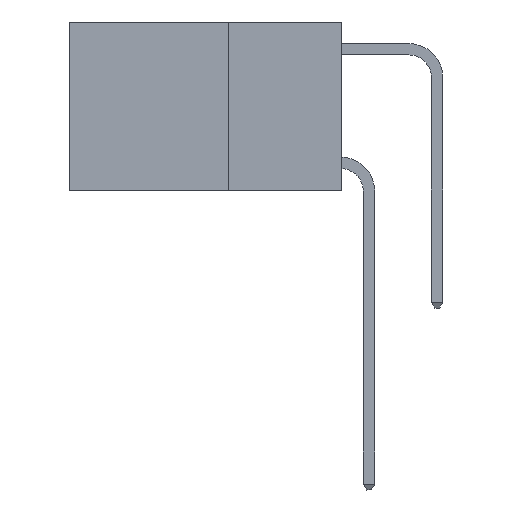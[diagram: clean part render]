
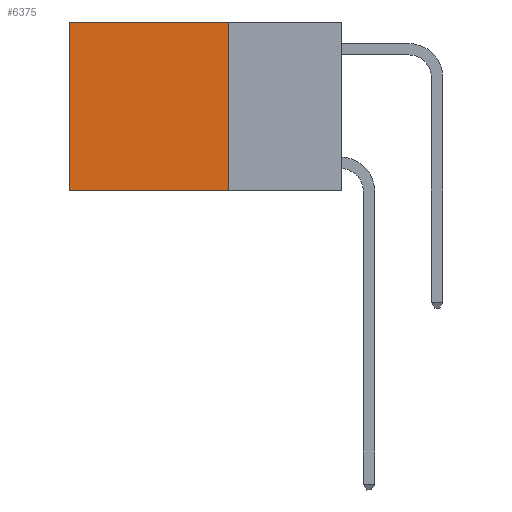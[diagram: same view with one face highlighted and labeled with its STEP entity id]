
A CAD part, left-side view. The second image highlights one B-rep face of the part: STEP entity #6375.
In plain terms, the highlighted planar face has unit normal (-1, 0, 0).
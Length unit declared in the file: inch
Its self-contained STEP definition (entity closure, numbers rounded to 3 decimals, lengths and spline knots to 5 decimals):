
#297 = CARTESIAN_POINT ( 'NONE',  ( 0.2625, 0.25, 0. ) ) ;
#798 = EDGE_CURVE ( 'NONE', #8440, #4409, #9333, .T. ) ;
#1024 = LINE ( 'NONE', #9739, #7808 ) ;
#1093 = DIRECTION ( 'NONE',  ( 0., 0., -1. ) ) ;
#1301 = DIRECTION ( 'NONE',  ( 1., 0., 0. ) ) ;
#1322 = LINE ( 'NONE', #11291, #12889 ) ;
#1547 = ORIENTED_EDGE ( 'NONE', *, *, #3289, .F. ) ;
#1710 = EDGE_LOOP ( 'NONE', ( #4981, #1547, #9969, #10829 ) ) ;
#3289 = EDGE_CURVE ( 'NONE', #4409, #6007, #1322, .T. ) ;
#3851 = DIRECTION ( 'NONE',  ( 0., 0., -1. ) ) ;
#3880 = LINE ( 'NONE', #4791, #10066 ) ;
#4409 = VERTEX_POINT ( 'NONE', #7246 ) ;
#4791 = CARTESIAN_POINT ( 'NONE',  ( 0.2625, 0.25, 0. ) ) ;
#4981 = ORIENTED_EDGE ( 'NONE', *, *, #6360, .T. ) ;
#5369 = DIRECTION ( 'NONE',  ( 0., 0., -1. ) ) ;
#5900 = CARTESIAN_POINT ( 'NONE',  ( 0.2625, 0.6, 0. ) ) ;
#6007 = VERTEX_POINT ( 'NONE', #8128 ) ;
#6360 = EDGE_CURVE ( 'NONE', #13377, #6007, #1024, .T. ) ;
#6375 = ADVANCED_FACE ( 'NONE', ( #11132 ), #6523, .F. ) ;
#6523 = PLANE ( 'NONE',  #11423 ) ;
#7055 = DIRECTION ( 'NONE',  ( 0., 1., 0. ) ) ;
#7246 = CARTESIAN_POINT ( 'NONE',  ( 0.2625, 0.25, -0.37 ) ) ;
#7407 = VECTOR ( 'NONE', #3851, 39.37008 ) ;
#7808 = VECTOR ( 'NONE', #5369, 39.37008 ) ;
#8128 = CARTESIAN_POINT ( 'NONE',  ( 0.2625, 0.6, -0.37 ) ) ;
#8145 = DIRECTION ( 'NONE',  ( 0., 1., 0. ) ) ;
#8440 = VERTEX_POINT ( 'NONE', #9616 ) ;
#9333 = LINE ( 'NONE', #13659, #7407 ) ;
#9616 = CARTESIAN_POINT ( 'NONE',  ( 0.2625, 0.25, 0. ) ) ;
#9739 = CARTESIAN_POINT ( 'NONE',  ( 0.2625, 0.6, 0. ) ) ;
#9969 = ORIENTED_EDGE ( 'NONE', *, *, #798, .F. ) ;
#10066 = VECTOR ( 'NONE', #8145, 39.37008 ) ;
#10829 = ORIENTED_EDGE ( 'NONE', *, *, #11661, .T. ) ;
#11132 = FACE_OUTER_BOUND ( 'NONE', #1710, .T. ) ;
#11291 = CARTESIAN_POINT ( 'NONE',  ( 0.2625, 0.25, -0.37 ) ) ;
#11423 = AXIS2_PLACEMENT_3D ( 'NONE', #297, #1301, #1093 ) ;
#11661 = EDGE_CURVE ( 'NONE', #8440, #13377, #3880, .T. ) ;
#12889 = VECTOR ( 'NONE', #7055, 39.37008 ) ;
#13377 = VERTEX_POINT ( 'NONE', #5900 ) ;
#13659 = CARTESIAN_POINT ( 'NONE',  ( 0.2625, 0.25, 0. ) ) ;
